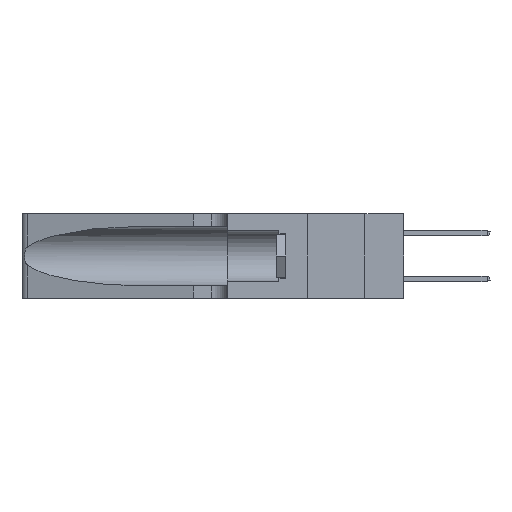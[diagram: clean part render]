
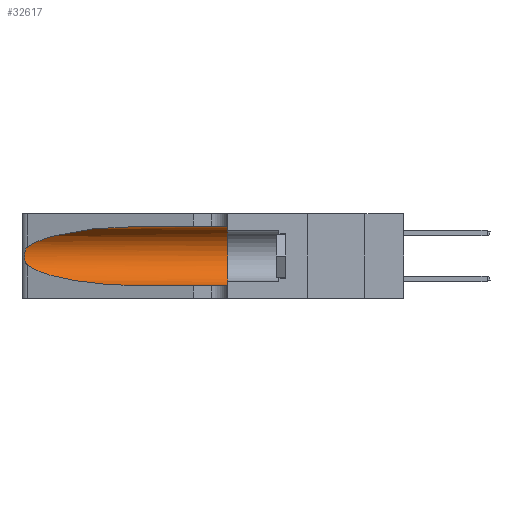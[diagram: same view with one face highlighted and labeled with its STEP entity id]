
A CAD part, left-side view. The second image highlights one B-rep face of the part: STEP entity #32617.
In plain terms, the highlighted cylindrical face has radius 3.308 mm (diameter 6.617 mm), a partial arc.
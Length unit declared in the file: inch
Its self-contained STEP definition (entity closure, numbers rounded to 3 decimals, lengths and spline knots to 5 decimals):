
#479 = CARTESIAN_POINT ( 'NONE',  ( 0.1305, 0.72297, 0.31525 ) ) ;
#1378 = B_SPLINE_CURVE_WITH_KNOTS ( 'NONE', 3,
 ( #15645, #35751, #21191, #4070, #12355, #9606, #12241, #20811, #18028, #12741, #3571, #15517, #9469, #21053 ),
 .UNSPECIFIED., .F., .F.,
 ( 4, 2, 2, 2, 2, 2, 4 ),
 ( 0., 0.00027, 0.00053, 0.00107, 0.0016, 0.00187, 0.00214 ),
 .UNSPECIFIED. ) ;
#2307 = VERTEX_POINT ( 'NONE', #7112 ) ;
#3312 = ORIENTED_EDGE ( 'NONE', *, *, #12495, .T. ) ;
#3571 = CARTESIAN_POINT ( 'NONE',  ( 0.25789, 1.23486, 0.15765 ) ) ;
#3916 = CARTESIAN_POINT ( 'NONE',  ( 0.1305, 1.61858, 0.05475 ) ) ;
#4070 = CARTESIAN_POINT ( 'NONE',  ( 0.25787, 1.23484, 0.2124 ) ) ;
#5054 = FACE_OUTER_BOUND ( 'NONE', #25869, .T. ) ;
#5788 = CARTESIAN_POINT ( 'NONE',  ( 0.1305, 0.35, 0.05475 ) ) ;
#5850 = ORIENTED_EDGE ( 'NONE', *, *, #28320, .F. ) ;
#6176 = CARTESIAN_POINT ( 'NONE',  ( 0.25487, 1.22718, 0.14631 ) ) ;
#7112 = CARTESIAN_POINT ( 'NONE',  ( 0.25487, 1.22718, 0.14631 ) ) ;
#7791 = DIRECTION ( 'NONE',  ( 0., 1., 0. ) ) ;
#8945 = CARTESIAN_POINT ( 'NONE',  ( 0.1305, 0.72297, 0.05475 ) ) ;
#9469 = CARTESIAN_POINT ( 'NONE',  ( 0.25555, 1.22993, 0.14849 ) ) ;
#9606 = CARTESIAN_POINT ( 'NONE',  ( 0.26018, 1.23835, 0.19895 ) ) ;
#10064 = CARTESIAN_POINT ( 'NONE',  ( 0.18966, 0.96281, 0.31525 ) ) ;
#12219 = AXIS2_PLACEMENT_3D ( 'NONE', #24541, #7791, #19000 ) ;
#12241 = CARTESIAN_POINT ( 'NONE',  ( 0.26075, 1.23896, 0.19203 ) ) ;
#12355 = CARTESIAN_POINT ( 'NONE',  ( 0.25854, 1.2359, 0.20912 ) ) ;
#12495 = EDGE_CURVE ( 'NONE', #16667, #30364, #36377, .T. ) ;
#12741 = CARTESIAN_POINT ( 'NONE',  ( 0.25856, 1.23593, 0.16098 ) ) ;
#12939 = EDGE_CURVE ( 'NONE', #16260, #27171, #34066, .T. ) ;
#14599 = CARTESIAN_POINT ( 'NONE',  ( 0.2373, 1.15595, 0.08982 ) ) ;
#14996 = DIRECTION ( 'NONE',  ( 0., -1., 0. ) ) ;
#15517 = CARTESIAN_POINT ( 'NONE',  ( 0.25639, 1.23186, 0.15144 ) ) ;
#15645 = CARTESIAN_POINT ( 'NONE',  ( 0.25487, 1.22718, 0.22369 ) ) ;
#16260 = VERTEX_POINT ( 'NONE', #479 ) ;
#16667 = VERTEX_POINT ( 'NONE', #19746 ) ;
#17493 = ORIENTED_EDGE ( 'NONE', *, *, #27396, .T. ) ;
#18028 = CARTESIAN_POINT ( 'NONE',  ( 0.26017, 1.23833, 0.17102 ) ) ;
#18455 = CARTESIAN_POINT ( 'NONE',  ( 0.25487, 1.22718, 0.22369 ) ) ;
#18771 = DIRECTION ( 'NONE',  ( 0., -1., 0. ) ) ;
#19000 = DIRECTION ( 'NONE',  ( 0., 0., 1. ) ) ;
#19035 = ORIENTED_EDGE ( 'NONE', *, *, #19676, .T. ) ;
#19298 = VECTOR ( 'NONE', #18771, 39.37008 ) ;
#19347 = CARTESIAN_POINT ( 'NONE',  ( 0.1305, 1.61858, 0.185 ) ) ;
#19676 = EDGE_CURVE ( 'NONE', #2307, #16667, #29229, .T. ) ;
#19746 = CARTESIAN_POINT ( 'NONE',  ( 0.1305, 0.72297, 0.05475 ) ) ;
#20811 = CARTESIAN_POINT ( 'NONE',  ( 0.26075, 1.23896, 0.178 ) ) ;
#21053 = CARTESIAN_POINT ( 'NONE',  ( 0.25487, 1.22718, 0.14631 ) ) ;
#21191 = CARTESIAN_POINT ( 'NONE',  ( 0.25639, 1.23184, 0.21858 ) ) ;
#22613 = CARTESIAN_POINT ( 'NONE',  ( 0.1305, 0.35, 0.31525 ) ) ;
#22853 = CARTESIAN_POINT ( 'NONE',  ( 0.1305, 1.61858, 0.31525 ) ) ;
#24541 = CARTESIAN_POINT ( 'NONE',  ( 0.1305, 0.35, 0.185 ) ) ;
#24670 = CARTESIAN_POINT ( 'NONE',  ( 0.25487, 1.22718, 0.22369 ) ) ;
#25869 = EDGE_LOOP ( 'NONE', ( #30300, #17493, #19035, #3312, #5850, #36701 ) ) ;
#25877 = DIRECTION ( 'NONE',  ( 0., 0., -1. ) ) ;
#26433 = VECTOR ( 'NONE', #14996, 39.37008 ) ;
#26440 = CARTESIAN_POINT ( 'NONE',  ( 0.18966, 0.96281, 0.05475 ) ) ;
#27171 = VERTEX_POINT ( 'NONE', #22613 ) ;
#27396 = EDGE_CURVE ( 'NONE', #32180, #2307, #1378, .T. ) ;
#28320 = EDGE_CURVE ( 'NONE', #27171, #30364, #33658, .T. ) ;
#29229 =( BOUNDED_CURVE ( )  B_SPLINE_CURVE ( 3, ( #6176, #14599, #26440, #8945 ),
 .UNSPECIFIED., .F., .T. ) 
 B_SPLINE_CURVE_WITH_KNOTS ( ( 4, 4 ),
 ( 3.44316, 4.71239 ),
 .UNSPECIFIED. ) 
 CURVE ( )  GEOMETRIC_REPRESENTATION_ITEM ( )  RATIONAL_B_SPLINE_CURVE ( ( 1., 0.87, 0.87, 1. ) ) 
 REPRESENTATION_ITEM ( '' )  );
#30300 = ORIENTED_EDGE ( 'NONE', *, *, #36155, .T. ) ;
#30364 = VERTEX_POINT ( 'NONE', #5788 ) ;
#31150 = AXIS2_PLACEMENT_3D ( 'NONE', #19347, #36927, #25877 ) ;
#31987 = CYLINDRICAL_SURFACE ( 'NONE', #31150, 0.13025 ) ;
#32180 = VERTEX_POINT ( 'NONE', #18455 ) ;
#32617 = ADVANCED_FACE ( 'NONE', ( #5054 ), #31987, .F. ) ;
#32681 =( BOUNDED_CURVE ( )  B_SPLINE_CURVE ( 3, ( #35835, #10064, #36328, #24670 ),
 .UNSPECIFIED., .F., .T. ) 
 B_SPLINE_CURVE_WITH_KNOTS ( ( 4, 4 ),
 ( 1.5708, 2.84003 ),
 .UNSPECIFIED. ) 
 CURVE ( )  GEOMETRIC_REPRESENTATION_ITEM ( )  RATIONAL_B_SPLINE_CURVE ( ( 1., 0.87, 0.87, 1. ) ) 
 REPRESENTATION_ITEM ( '' )  );
#33658 = CIRCLE ( 'NONE', #12219, 0.13025 ) ;
#34066 = LINE ( 'NONE', #22853, #26433 ) ;
#35751 = CARTESIAN_POINT ( 'NONE',  ( 0.25555, 1.22994, 0.2215 ) ) ;
#35835 = CARTESIAN_POINT ( 'NONE',  ( 0.1305, 0.72297, 0.31525 ) ) ;
#36155 = EDGE_CURVE ( 'NONE', #16260, #32180, #32681, .T. ) ;
#36328 = CARTESIAN_POINT ( 'NONE',  ( 0.2373, 1.15595, 0.28018 ) ) ;
#36377 = LINE ( 'NONE', #3916, #19298 ) ;
#36701 = ORIENTED_EDGE ( 'NONE', *, *, #12939, .F. ) ;
#36927 = DIRECTION ( 'NONE',  ( 0., -1., 0. ) ) ;
